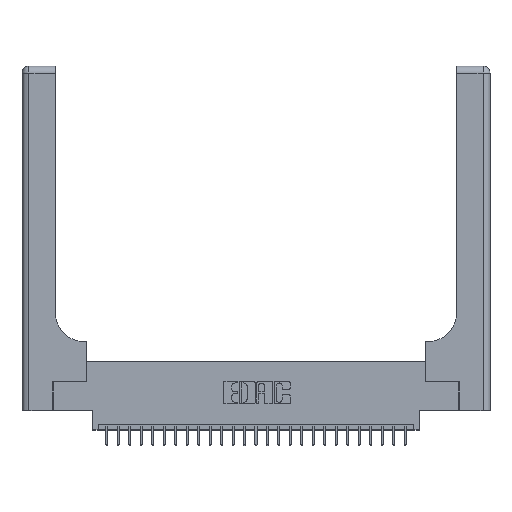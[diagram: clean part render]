
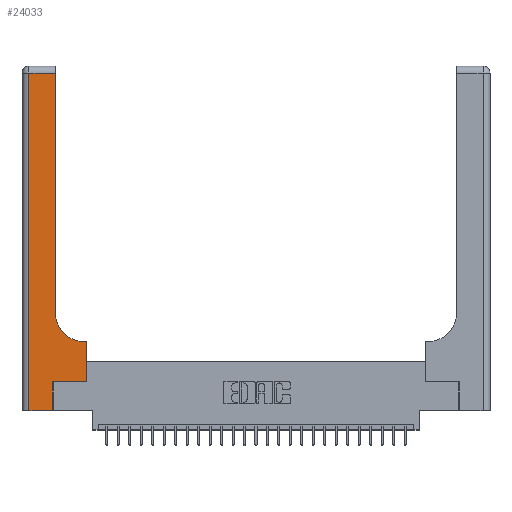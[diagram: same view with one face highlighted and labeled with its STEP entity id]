
A CAD part, top view. The second image highlights one B-rep face of the part: STEP entity #24033.
In plain terms, the highlighted planar face has unit normal (0, 0, 1).
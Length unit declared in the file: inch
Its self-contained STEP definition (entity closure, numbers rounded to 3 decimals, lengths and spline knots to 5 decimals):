
#307 = CARTESIAN_POINT ( 'NONE',  ( 0.269, 0.25, 0.37 ) ) ;
#518 = VECTOR ( 'NONE', #18777, 39.37008 ) ;
#742 = VERTEX_POINT ( 'NONE', #12809 ) ;
#1288 = LINE ( 'NONE', #7993, #23233 ) ;
#1559 = CARTESIAN_POINT ( 'NONE',  ( 0.06, 0., 0.37 ) ) ;
#2130 = DIRECTION ( 'NONE',  ( 1., 0., 0. ) ) ;
#2265 = VERTEX_POINT ( 'NONE', #27764 ) ;
#3468 = CARTESIAN_POINT ( 'NONE',  ( 0.5415, 0.6, 0.37 ) ) ;
#3575 = LINE ( 'NONE', #5748, #518 ) ;
#3760 = VECTOR ( 'NONE', #15034, 39.37008 ) ;
#3934 = ORIENTED_EDGE ( 'NONE', *, *, #17968, .T. ) ;
#4745 = ORIENTED_EDGE ( 'NONE', *, *, #19822, .T. ) ;
#4887 = VERTEX_POINT ( 'NONE', #25850 ) ;
#5748 = CARTESIAN_POINT ( 'NONE',  ( 0.269, 0.25, 0.37 ) ) ;
#6296 = EDGE_CURVE ( 'NONE', #7518, #2265, #24537, .T. ) ;
#6525 = DIRECTION ( 'NONE',  ( 0., 0., -1. ) ) ;
#6646 = LINE ( 'NONE', #15473, #24629 ) ;
#7299 = EDGE_CURVE ( 'NONE', #2265, #17677, #17622, .T. ) ;
#7409 = EDGE_CURVE ( 'NONE', #11136, #14993, #6646, .T. ) ;
#7518 = VERTEX_POINT ( 'NONE', #1559 ) ;
#7529 = LINE ( 'NONE', #9551, #10679 ) ;
#7968 = ORIENTED_EDGE ( 'NONE', *, *, #7299, .T. ) ;
#7993 = CARTESIAN_POINT ( 'NONE',  ( 0.5585, 0.25, 0.37 ) ) ;
#8124 = EDGE_CURVE ( 'NONE', #4887, #7518, #27924, .T. ) ;
#8266 = DIRECTION ( 'NONE',  ( 0., -1., 0. ) ) ;
#8675 = CARTESIAN_POINT ( 'NONE',  ( 0.269, 0., 0.37 ) ) ;
#8683 = AXIS2_PLACEMENT_3D ( 'NONE', #17640, #6525, #2130 ) ;
#9551 = CARTESIAN_POINT ( 'NONE',  ( 0.2915, 3., 0.37 ) ) ;
#9575 = LINE ( 'NONE', #18652, #15489 ) ;
#9860 = DIRECTION ( 'NONE',  ( -1., 0., 0. ) ) ;
#10316 = EDGE_LOOP ( 'NONE', ( #16493, #4745, #21812, #11020, #7968, #16697, #3934, #12646, #12290 ) ) ;
#10679 = VECTOR ( 'NONE', #27038, 39.37008 ) ;
#11020 = ORIENTED_EDGE ( 'NONE', *, *, #6296, .T. ) ;
#11124 = DIRECTION ( 'NONE',  ( 1., 0., 0. ) ) ;
#11136 = VERTEX_POINT ( 'NONE', #20852 ) ;
#11933 = CIRCLE ( 'NONE', #8683, 0.25 ) ;
#12290 = ORIENTED_EDGE ( 'NONE', *, *, #21459, .T. ) ;
#12328 = AXIS2_PLACEMENT_3D ( 'NONE', #19402, #22163, #17809 ) ;
#12618 = EDGE_CURVE ( 'NONE', #17883, #12902, #7529, .T. ) ;
#12646 = ORIENTED_EDGE ( 'NONE', *, *, #7409, .T. ) ;
#12809 = CARTESIAN_POINT ( 'NONE',  ( 0.5585, 0.25, 0.37 ) ) ;
#12902 = VERTEX_POINT ( 'NONE', #28022 ) ;
#13562 = CARTESIAN_POINT ( 'NONE',  ( 0., 0., 0.37 ) ) ;
#13965 = EDGE_CURVE ( 'NONE', #17677, #742, #3575, .T. ) ;
#14993 = VERTEX_POINT ( 'NONE', #3468 ) ;
#15034 = DIRECTION ( 'NONE',  ( 0., 1., 0. ) ) ;
#15090 = FACE_OUTER_BOUND ( 'NONE', #10316, .T. ) ;
#15473 = CARTESIAN_POINT ( 'NONE',  ( 0.2915, 0.6, 0.37 ) ) ;
#15489 = VECTOR ( 'NONE', #9860, 39.37008 ) ;
#16493 = ORIENTED_EDGE ( 'NONE', *, *, #12618, .T. ) ;
#16664 = DIRECTION ( 'NONE',  ( 0., 1., 0. ) ) ;
#16697 = ORIENTED_EDGE ( 'NONE', *, *, #13965, .T. ) ;
#17622 = LINE ( 'NONE', #8675, #3760 ) ;
#17640 = CARTESIAN_POINT ( 'NONE',  ( 0.5415, 0.85, 0.37 ) ) ;
#17677 = VERTEX_POINT ( 'NONE', #307 ) ;
#17809 = DIRECTION ( 'NONE',  ( -1., 0., 0. ) ) ;
#17883 = VERTEX_POINT ( 'NONE', #25340 ) ;
#17968 = EDGE_CURVE ( 'NONE', #742, #11136, #1288, .T. ) ;
#18411 = VECTOR ( 'NONE', #11124, 39.37008 ) ;
#18652 = CARTESIAN_POINT ( 'NONE',  ( 0., 2.94, 0.37 ) ) ;
#18777 = DIRECTION ( 'NONE',  ( 1., 0., 0. ) ) ;
#19402 = CARTESIAN_POINT ( 'NONE',  ( 0., 3., 0.37 ) ) ;
#19822 = EDGE_CURVE ( 'NONE', #12902, #4887, #9575, .T. ) ;
#20852 = CARTESIAN_POINT ( 'NONE',  ( 0.5585, 0.6, 0.37 ) ) ;
#21459 = EDGE_CURVE ( 'NONE', #14993, #17883, #11933, .T. ) ;
#21812 = ORIENTED_EDGE ( 'NONE', *, *, #8124, .T. ) ;
#22163 = DIRECTION ( 'NONE',  ( 0., 0., -1. ) ) ;
#23233 = VECTOR ( 'NONE', #16664, 39.37008 ) ;
#23885 = PLANE ( 'NONE',  #12328 ) ;
#24033 = ADVANCED_FACE ( 'NONE', ( #15090 ), #23885, .F. ) ;
#24272 = DIRECTION ( 'NONE',  ( -1., 0., 0. ) ) ;
#24395 = VECTOR ( 'NONE', #8266, 39.37008 ) ;
#24537 = LINE ( 'NONE', #13562, #18411 ) ;
#24629 = VECTOR ( 'NONE', #24272, 39.37008 ) ;
#25340 = CARTESIAN_POINT ( 'NONE',  ( 0.2915, 0.85, 0.37 ) ) ;
#25850 = CARTESIAN_POINT ( 'NONE',  ( 0.06, 2.94, 0.37 ) ) ;
#27038 = DIRECTION ( 'NONE',  ( 0., 1., 0. ) ) ;
#27764 = CARTESIAN_POINT ( 'NONE',  ( 0.269, 0., 0.37 ) ) ;
#27924 = LINE ( 'NONE', #28221, #24395 ) ;
#28022 = CARTESIAN_POINT ( 'NONE',  ( 0.2915, 2.94, 0.37 ) ) ;
#28221 = CARTESIAN_POINT ( 'NONE',  ( 0.06, 3., 0.37 ) ) ;
